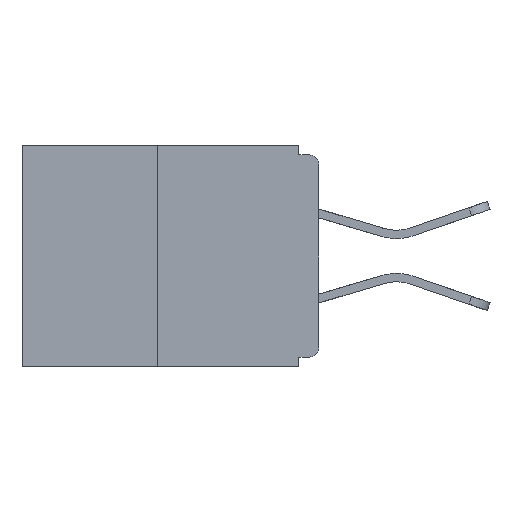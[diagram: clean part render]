
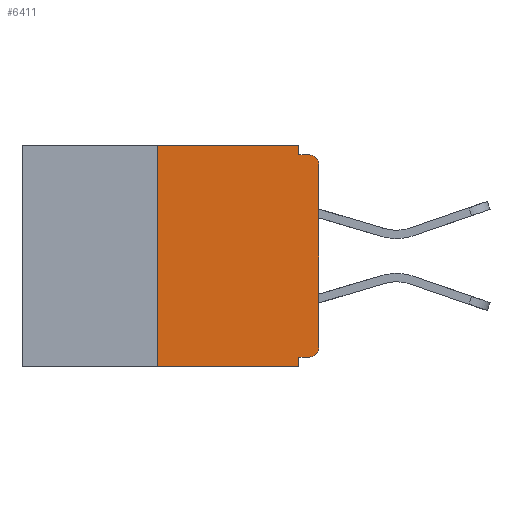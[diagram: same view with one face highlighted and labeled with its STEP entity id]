
A CAD part, left-side view. The second image highlights one B-rep face of the part: STEP entity #6411.
In plain terms, the highlighted planar face has unit normal (-1, 0, 0).
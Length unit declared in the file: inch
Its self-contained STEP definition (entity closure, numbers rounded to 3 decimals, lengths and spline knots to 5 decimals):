
#114 = EDGE_CURVE ( 'NONE', #4096, #1702, #4672, .T. ) ;
#723 = PLANE ( 'NONE',  #5715 ) ;
#1125 = ORIENTED_EDGE ( 'NONE', *, *, #4041, .F. ) ;
#1190 = VECTOR ( 'NONE', #10371, 39.37008 ) ;
#1193 = ORIENTED_EDGE ( 'NONE', *, *, #10310, .F. ) ;
#1318 = VERTEX_POINT ( 'NONE', #4056 ) ;
#1458 = ORIENTED_EDGE ( 'NONE', *, *, #6806, .F. ) ;
#1577 = CARTESIAN_POINT ( 'NONE',  ( 0., 0.25, 0. ) ) ;
#1591 = DIRECTION ( 'NONE',  ( 0., -1., 0. ) ) ;
#1592 = CARTESIAN_POINT ( 'NONE',  ( 0., 0.031, 0. ) ) ;
#1689 = VERTEX_POINT ( 'NONE', #6782 ) ;
#1702 = VERTEX_POINT ( 'NONE', #5027 ) ;
#1790 = EDGE_CURVE ( 'NONE', #1318, #8368, #4906, .T. ) ;
#1906 = VECTOR ( 'NONE', #10044, 39.37008 ) ;
#1978 = FACE_OUTER_BOUND ( 'NONE', #9020, .T. ) ;
#2147 = CARTESIAN_POINT ( 'NONE',  ( 0., 0.46, -0.343 ) ) ;
#2162 = DIRECTION ( 'NONE',  ( 0., 0., -1. ) ) ;
#2228 = VERTEX_POINT ( 'NONE', #2287 ) ;
#2287 = CARTESIAN_POINT ( 'NONE',  ( 0., 0.031, -0.343 ) ) ;
#2387 = LINE ( 'NONE', #1577, #4907 ) ;
#2533 = CARTESIAN_POINT ( 'NONE',  ( 0., 0.46, 0. ) ) ;
#2571 = DIRECTION ( 'NONE',  ( 1., 0., 0. ) ) ;
#2623 = ORIENTED_EDGE ( 'NONE', *, *, #7146, .F. ) ;
#2683 = DIRECTION ( 'NONE',  ( 0., 0., -1. ) ) ;
#2741 = ORIENTED_EDGE ( 'NONE', *, *, #6449, .T. ) ;
#2892 = DIRECTION ( 'NONE',  ( 0., -1., 0. ) ) ;
#3167 = LINE ( 'NONE', #3621, #5266 ) ;
#3316 = CIRCLE ( 'NONE', #6968, 0.015 ) ;
#3599 = CARTESIAN_POINT ( 'NONE',  ( 0., 0., -0.313 ) ) ;
#3605 = EDGE_CURVE ( 'NONE', #3914, #4091, #3167, .T. ) ;
#3620 = LINE ( 'NONE', #4747, #9890 ) ;
#3621 = CARTESIAN_POINT ( 'NONE',  ( 0., 0.46, 0. ) ) ;
#3748 = CARTESIAN_POINT ( 'NONE',  ( 0., 0.015, -0.015 ) ) ;
#3914 = VERTEX_POINT ( 'NONE', #4921 ) ;
#4041 = EDGE_CURVE ( 'NONE', #4091, #1318, #5822, .T. ) ;
#4056 = CARTESIAN_POINT ( 'NONE',  ( 0., 0.031, -0.015 ) ) ;
#4091 = VERTEX_POINT ( 'NONE', #5208 ) ;
#4096 = VERTEX_POINT ( 'NONE', #3599 ) ;
#4098 = EDGE_CURVE ( 'NONE', #6808, #4096, #3316, .T. ) ;
#4554 = LINE ( 'NONE', #2147, #1906 ) ;
#4672 = LINE ( 'NONE', #5277, #8849 ) ;
#4746 = CARTESIAN_POINT ( 'NONE',  ( 0., 0.015, -0.313 ) ) ;
#4747 = CARTESIAN_POINT ( 'NONE',  ( 0., 0.031, -0.343 ) ) ;
#4861 = DIRECTION ( 'NONE',  ( 0., 0., -1. ) ) ;
#4906 = LINE ( 'NONE', #7004, #6153 ) ;
#4907 = VECTOR ( 'NONE', #7810, 39.37008 ) ;
#4921 = CARTESIAN_POINT ( 'NONE',  ( 0., 0.25, 0. ) ) ;
#5027 = CARTESIAN_POINT ( 'NONE',  ( 0., 0., -0.03 ) ) ;
#5208 = CARTESIAN_POINT ( 'NONE',  ( 0., 0.031, 0. ) ) ;
#5266 = VECTOR ( 'NONE', #2892, 39.37008 ) ;
#5277 = CARTESIAN_POINT ( 'NONE',  ( 0., 0., 0. ) ) ;
#5319 = DIRECTION ( 'NONE',  ( 0., 0., -1. ) ) ;
#5715 = AXIS2_PLACEMENT_3D ( 'NONE', #2533, #2571, #5319 ) ;
#5822 = LINE ( 'NONE', #1592, #10709 ) ;
#5932 = CARTESIAN_POINT ( 'NONE',  ( 0., 0., -0.328 ) ) ;
#5977 = ORIENTED_EDGE ( 'NONE', *, *, #3605, .F. ) ;
#6153 = VECTOR ( 'NONE', #1591, 39.37008 ) ;
#6335 = ORIENTED_EDGE ( 'NONE', *, *, #11128, .T. ) ;
#6411 = ADVANCED_FACE ( 'NONE', ( #1978 ), #723, .F. ) ;
#6449 = EDGE_CURVE ( 'NONE', #1702, #8368, #8656, .T. ) ;
#6599 = DIRECTION ( 'NONE',  ( -1., 0., 0. ) ) ;
#6782 = CARTESIAN_POINT ( 'NONE',  ( 0., 0.25, -0.343 ) ) ;
#6806 = EDGE_CURVE ( 'NONE', #1689, #3914, #2387, .T. ) ;
#6808 = VERTEX_POINT ( 'NONE', #6925 ) ;
#6856 = ORIENTED_EDGE ( 'NONE', *, *, #4098, .T. ) ;
#6925 = CARTESIAN_POINT ( 'NONE',  ( 0., 0.015, -0.328 ) ) ;
#6968 = AXIS2_PLACEMENT_3D ( 'NONE', #4746, #6599, #2162 ) ;
#7004 = CARTESIAN_POINT ( 'NONE',  ( 0., 0., -0.015 ) ) ;
#7006 = CARTESIAN_POINT ( 'NONE',  ( 0., 0.015, -0.03 ) ) ;
#7146 = EDGE_CURVE ( 'NONE', #10245, #2228, #3620, .T. ) ;
#7508 = CARTESIAN_POINT ( 'NONE',  ( 0., 0.031, -0.328 ) ) ;
#7810 = DIRECTION ( 'NONE',  ( 0., 0., 1. ) ) ;
#7947 = DIRECTION ( 'NONE',  ( -1., 0., 0. ) ) ;
#8368 = VERTEX_POINT ( 'NONE', #3748 ) ;
#8383 = ORIENTED_EDGE ( 'NONE', *, *, #1790, .F. ) ;
#8656 = CIRCLE ( 'NONE', #10105, 0.015 ) ;
#8849 = VECTOR ( 'NONE', #11487, 39.37008 ) ;
#8896 = ORIENTED_EDGE ( 'NONE', *, *, #114, .T. ) ;
#9020 = EDGE_LOOP ( 'NONE', ( #5977, #1458, #6335, #2623, #1193, #6856, #8896, #2741, #8383, #1125 ) ) ;
#9582 = DIRECTION ( 'NONE',  ( 0., 0., -1. ) ) ;
#9815 = LINE ( 'NONE', #5932, #1190 ) ;
#9890 = VECTOR ( 'NONE', #4861, 39.37008 ) ;
#10044 = DIRECTION ( 'NONE',  ( 0., -1., 0. ) ) ;
#10105 = AXIS2_PLACEMENT_3D ( 'NONE', #7006, #7947, #2683 ) ;
#10245 = VERTEX_POINT ( 'NONE', #7508 ) ;
#10310 = EDGE_CURVE ( 'NONE', #6808, #10245, #9815, .T. ) ;
#10371 = DIRECTION ( 'NONE',  ( 0., 1., 0. ) ) ;
#10709 = VECTOR ( 'NONE', #9582, 39.37008 ) ;
#11128 = EDGE_CURVE ( 'NONE', #1689, #2228, #4554, .T. ) ;
#11487 = DIRECTION ( 'NONE',  ( 0., 0., 1. ) ) ;
